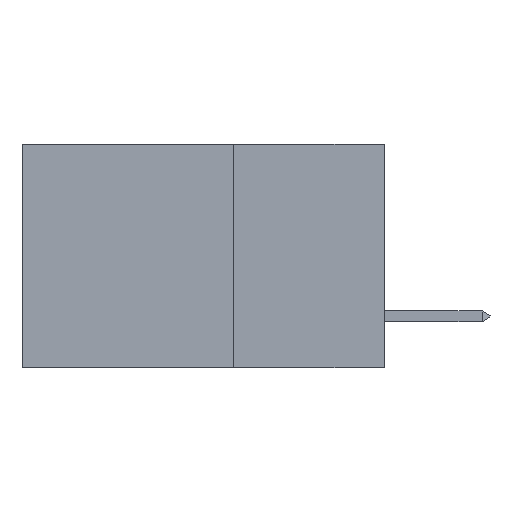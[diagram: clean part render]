
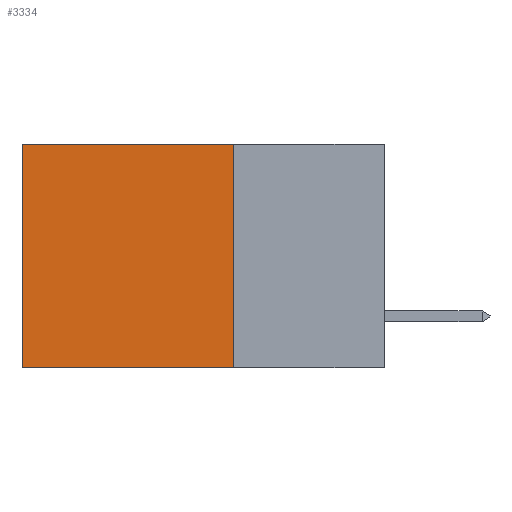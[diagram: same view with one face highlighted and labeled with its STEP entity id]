
A CAD part, left-side view. The second image highlights one B-rep face of the part: STEP entity #3334.
In plain terms, the highlighted planar face has unit normal (-1, 0, 0).
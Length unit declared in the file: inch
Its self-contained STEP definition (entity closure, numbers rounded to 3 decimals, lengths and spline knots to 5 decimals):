
#797 = LINE ( 'NONE', #16182, #27054 ) ;
#1202 = AXIS2_PLACEMENT_3D ( 'NONE', #18187, #15892, #4959 ) ;
#1614 = VECTOR ( 'NONE', #2868, 39.37008 ) ;
#2091 = DIRECTION ( 'NONE',  ( 0., 0., -1. ) ) ;
#2868 = DIRECTION ( 'NONE',  ( 0., 1., 0. ) ) ;
#3081 = FACE_OUTER_BOUND ( 'NONE', #16428, .T. ) ;
#3119 = EDGE_CURVE ( 'NONE', #26150, #26599, #19933, .T. ) ;
#3334 = ADVANCED_FACE ( 'NONE', ( #3081 ), #20650, .F. ) ;
#4612 = LINE ( 'NONE', #13390, #18765 ) ;
#4894 = LINE ( 'NONE', #18543, #1614 ) ;
#4959 = DIRECTION ( 'NONE',  ( 0., 0., -1. ) ) ;
#5950 = CARTESIAN_POINT ( 'NONE',  ( 0.2875, 0.6, 0. ) ) ;
#7551 = DIRECTION ( 'NONE',  ( 0., 0., -1. ) ) ;
#9383 = EDGE_CURVE ( 'NONE', #26599, #25573, #4612, .T. ) ;
#10612 = ORIENTED_EDGE ( 'NONE', *, *, #21028, .T. ) ;
#11789 = VERTEX_POINT ( 'NONE', #5950 ) ;
#12569 = ORIENTED_EDGE ( 'NONE', *, *, #9383, .F. ) ;
#13390 = CARTESIAN_POINT ( 'NONE',  ( 0.2875, 0.25, -0.37 ) ) ;
#13828 = ORIENTED_EDGE ( 'NONE', *, *, #24350, .T. ) ;
#15892 = DIRECTION ( 'NONE',  ( 1., 0., 0. ) ) ;
#16182 = CARTESIAN_POINT ( 'NONE',  ( 0.2875, 0.6, 0. ) ) ;
#16428 = EDGE_LOOP ( 'NONE', ( #13828, #12569, #26969, #10612 ) ) ;
#17779 = CARTESIAN_POINT ( 'NONE',  ( 0.2875, 0.25, 0. ) ) ;
#18187 = CARTESIAN_POINT ( 'NONE',  ( 0.2875, 0.25, 0. ) ) ;
#18543 = CARTESIAN_POINT ( 'NONE',  ( 0.2875, 0.25, 0. ) ) ;
#18765 = VECTOR ( 'NONE', #19996, 39.37008 ) ;
#19219 = VECTOR ( 'NONE', #2091, 39.37008 ) ;
#19933 = LINE ( 'NONE', #17779, #19219 ) ;
#19996 = DIRECTION ( 'NONE',  ( 0., 1., 0. ) ) ;
#20650 = PLANE ( 'NONE',  #1202 ) ;
#21028 = EDGE_CURVE ( 'NONE', #26150, #11789, #4894, .T. ) ;
#22404 = CARTESIAN_POINT ( 'NONE',  ( 0.2875, 0.6, -0.37 ) ) ;
#22484 = CARTESIAN_POINT ( 'NONE',  ( 0.2875, 0.25, -0.37 ) ) ;
#24350 = EDGE_CURVE ( 'NONE', #11789, #25573, #797, .T. ) ;
#24528 = CARTESIAN_POINT ( 'NONE',  ( 0.2875, 0.25, 0. ) ) ;
#25573 = VERTEX_POINT ( 'NONE', #22404 ) ;
#26150 = VERTEX_POINT ( 'NONE', #24528 ) ;
#26599 = VERTEX_POINT ( 'NONE', #22484 ) ;
#26969 = ORIENTED_EDGE ( 'NONE', *, *, #3119, .F. ) ;
#27054 = VECTOR ( 'NONE', #7551, 39.37008 ) ;
